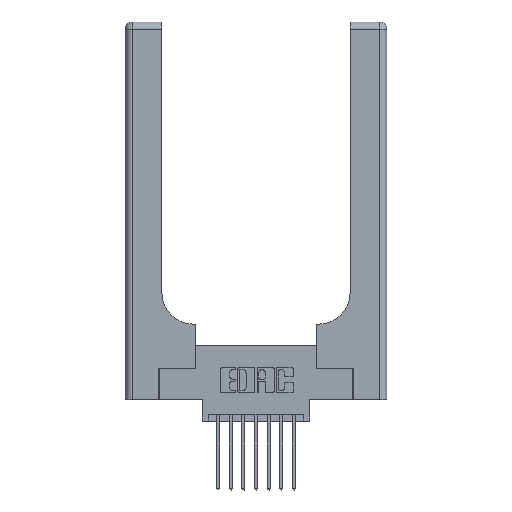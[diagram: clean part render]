
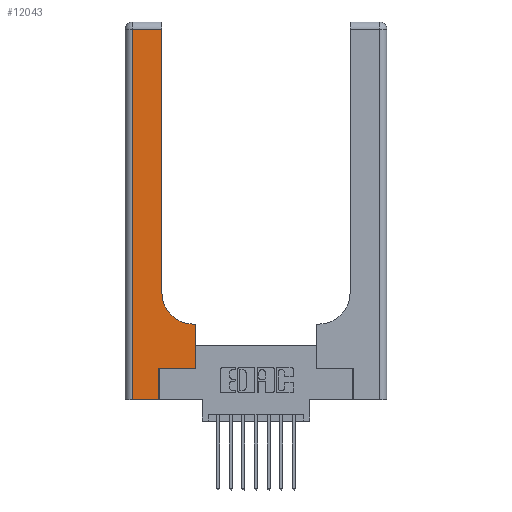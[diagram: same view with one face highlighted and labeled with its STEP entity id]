
A CAD part, top view. The second image highlights one B-rep face of the part: STEP entity #12043.
In plain terms, the highlighted planar face has unit normal (0, 0, 1).
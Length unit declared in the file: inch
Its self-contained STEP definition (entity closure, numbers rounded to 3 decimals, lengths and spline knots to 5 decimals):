
#571 = EDGE_CURVE ( 'NONE', #7057, #8103, #2803, .T. ) ;
#843 = VECTOR ( 'NONE', #14012, 39.37008 ) ;
#885 = DIRECTION ( 'NONE',  ( 0., 1., 0. ) ) ;
#1117 = CARTESIAN_POINT ( 'NONE',  ( 0.5415, 0.85, 0.37 ) ) ;
#1163 = ORIENTED_EDGE ( 'NONE', *, *, #15085, .T. ) ;
#1411 = DIRECTION ( 'NONE',  ( -1., 0., 0. ) ) ;
#1537 = EDGE_CURVE ( 'NONE', #1659, #5762, #6776, .T. ) ;
#1558 = CARTESIAN_POINT ( 'NONE',  ( 0.269, 0.25, 0.37 ) ) ;
#1643 = ORIENTED_EDGE ( 'NONE', *, *, #12247, .T. ) ;
#1659 = VERTEX_POINT ( 'NONE', #4421 ) ;
#2050 = ORIENTED_EDGE ( 'NONE', *, *, #10998, .T. ) ;
#2203 = CARTESIAN_POINT ( 'NONE',  ( 0.5415, 0.6, 0.37 ) ) ;
#2379 = DIRECTION ( 'NONE',  ( 1., 0., 0. ) ) ;
#2803 = LINE ( 'NONE', #13000, #6049 ) ;
#3136 = CARTESIAN_POINT ( 'NONE',  ( 0.269, 0., 0.37 ) ) ;
#3247 = EDGE_CURVE ( 'NONE', #5762, #14285, #6719, .T. ) ;
#3248 = VECTOR ( 'NONE', #885, 39.37008 ) ;
#3693 = VECTOR ( 'NONE', #12145, 39.37008 ) ;
#3827 = VERTEX_POINT ( 'NONE', #1558 ) ;
#4090 = LINE ( 'NONE', #4988, #3693 ) ;
#4098 = CARTESIAN_POINT ( 'NONE',  ( 0., 2.94, 0.37 ) ) ;
#4224 = LINE ( 'NONE', #4098, #10613 ) ;
#4421 = CARTESIAN_POINT ( 'NONE',  ( 0.5585, 0.25, 0.37 ) ) ;
#4812 = CARTESIAN_POINT ( 'NONE',  ( 0.06, 2.94, 0.37 ) ) ;
#4880 = DIRECTION ( 'NONE',  ( 0., 1., 0. ) ) ;
#4910 = CARTESIAN_POINT ( 'NONE',  ( 0.5585, 0.25, 0.37 ) ) ;
#4988 = CARTESIAN_POINT ( 'NONE',  ( 0.2915, 3., 0.37 ) ) ;
#5398 = CARTESIAN_POINT ( 'NONE',  ( 0., 3., 0.37 ) ) ;
#5534 = ORIENTED_EDGE ( 'NONE', *, *, #10690, .T. ) ;
#5762 = VERTEX_POINT ( 'NONE', #7881 ) ;
#5792 = AXIS2_PLACEMENT_3D ( 'NONE', #5398, #13745, #6658 ) ;
#6049 = VECTOR ( 'NONE', #12904, 39.37008 ) ;
#6223 = ORIENTED_EDGE ( 'NONE', *, *, #13135, .T. ) ;
#6331 = VERTEX_POINT ( 'NONE', #6740 ) ;
#6658 = DIRECTION ( 'NONE',  ( -1., 0., 0. ) ) ;
#6719 = LINE ( 'NONE', #7514, #12671 ) ;
#6740 = CARTESIAN_POINT ( 'NONE',  ( 0.2915, 2.94, 0.37 ) ) ;
#6776 = LINE ( 'NONE', #4910, #12722 ) ;
#6884 = CARTESIAN_POINT ( 'NONE',  ( 0.06, 0., 0.37 ) ) ;
#7008 = CARTESIAN_POINT ( 'NONE',  ( 0.269, 0., 0.37 ) ) ;
#7057 = VERTEX_POINT ( 'NONE', #6884 ) ;
#7514 = CARTESIAN_POINT ( 'NONE',  ( 0.2915, 0.6, 0.37 ) ) ;
#7651 = VERTEX_POINT ( 'NONE', #10509 ) ;
#7881 = CARTESIAN_POINT ( 'NONE',  ( 0.5585, 0.6, 0.37 ) ) ;
#8103 = VERTEX_POINT ( 'NONE', #3136 ) ;
#9641 = DIRECTION ( 'NONE',  ( 0., 0., -1. ) ) ;
#9666 = DIRECTION ( 'NONE',  ( 1., 0., 0. ) ) ;
#10028 = ORIENTED_EDGE ( 'NONE', *, *, #3247, .T. ) ;
#10191 = CIRCLE ( 'NONE', #14504, 0.25 ) ;
#10509 = CARTESIAN_POINT ( 'NONE',  ( 0.2915, 0.85, 0.37 ) ) ;
#10537 = LINE ( 'NONE', #12855, #843 ) ;
#10613 = VECTOR ( 'NONE', #12480, 39.37008 ) ;
#10690 = EDGE_CURVE ( 'NONE', #6331, #13822, #4224, .T. ) ;
#10713 = VECTOR ( 'NONE', #9666, 39.37008 ) ;
#10998 = EDGE_CURVE ( 'NONE', #8103, #3827, #12808, .T. ) ;
#11408 = PLANE ( 'NONE',  #5792 ) ;
#12034 = ORIENTED_EDGE ( 'NONE', *, *, #1537, .T. ) ;
#12043 = ADVANCED_FACE ( 'NONE', ( #15484 ), #11408, .F. ) ;
#12145 = DIRECTION ( 'NONE',  ( 0., 1., 0. ) ) ;
#12247 = EDGE_CURVE ( 'NONE', #14285, #7651, #10191, .T. ) ;
#12480 = DIRECTION ( 'NONE',  ( -1., 0., 0. ) ) ;
#12576 = EDGE_LOOP ( 'NONE', ( #1163, #5534, #6223, #14057, #2050, #14229, #12034, #10028, #1643 ) ) ;
#12671 = VECTOR ( 'NONE', #1411, 39.37008 ) ;
#12722 = VECTOR ( 'NONE', #4880, 39.37008 ) ;
#12808 = LINE ( 'NONE', #7008, #3248 ) ;
#12855 = CARTESIAN_POINT ( 'NONE',  ( 0.06, 3., 0.37 ) ) ;
#12904 = DIRECTION ( 'NONE',  ( 1., 0., 0. ) ) ;
#13000 = CARTESIAN_POINT ( 'NONE',  ( 0., 0., 0.37 ) ) ;
#13135 = EDGE_CURVE ( 'NONE', #13822, #7057, #10537, .T. ) ;
#13150 = CARTESIAN_POINT ( 'NONE',  ( 0.269, 0.25, 0.37 ) ) ;
#13352 = EDGE_CURVE ( 'NONE', #3827, #1659, #13823, .T. ) ;
#13745 = DIRECTION ( 'NONE',  ( 0., 0., -1. ) ) ;
#13822 = VERTEX_POINT ( 'NONE', #4812 ) ;
#13823 = LINE ( 'NONE', #13150, #10713 ) ;
#14012 = DIRECTION ( 'NONE',  ( 0., -1., 0. ) ) ;
#14057 = ORIENTED_EDGE ( 'NONE', *, *, #571, .T. ) ;
#14229 = ORIENTED_EDGE ( 'NONE', *, *, #13352, .T. ) ;
#14285 = VERTEX_POINT ( 'NONE', #2203 ) ;
#14504 = AXIS2_PLACEMENT_3D ( 'NONE', #1117, #9641, #2379 ) ;
#15085 = EDGE_CURVE ( 'NONE', #7651, #6331, #4090, .T. ) ;
#15484 = FACE_OUTER_BOUND ( 'NONE', #12576, .T. ) ;
